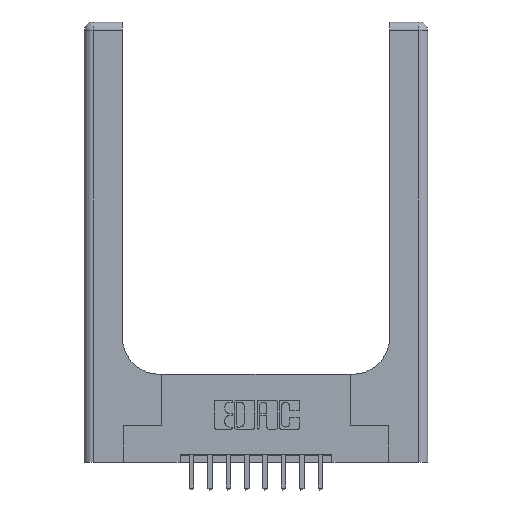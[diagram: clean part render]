
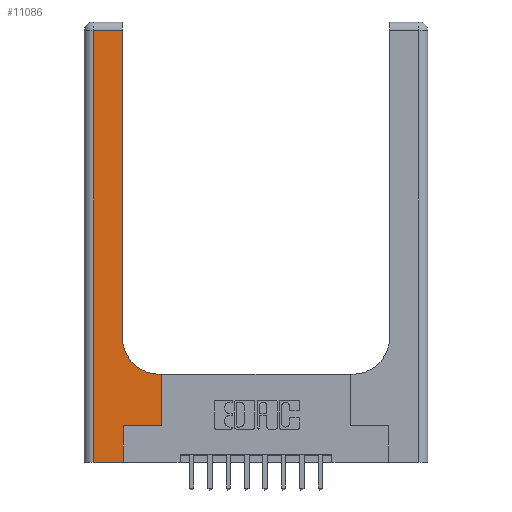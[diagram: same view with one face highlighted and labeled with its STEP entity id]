
A CAD part, top view. The second image highlights one B-rep face of the part: STEP entity #11086.
In plain terms, the highlighted planar face has unit normal (0, 0, 1).
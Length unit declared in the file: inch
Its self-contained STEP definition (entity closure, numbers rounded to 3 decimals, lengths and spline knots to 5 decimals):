
#569 = PLANE ( 'NONE',  #2759 ) ;
#762 = VECTOR ( 'NONE', #5868, 39.37008 ) ;
#809 = VECTOR ( 'NONE', #9433, 39.37008 ) ;
#1351 = EDGE_CURVE ( 'NONE', #14133, #10040, #5697, .T. ) ;
#1452 = CARTESIAN_POINT ( 'NONE',  ( 0., 2.94, 0.37 ) ) ;
#1755 = FACE_OUTER_BOUND ( 'NONE', #10992, .T. ) ;
#1768 = AXIS2_PLACEMENT_3D ( 'NONE', #4816, #14086, #13074 ) ;
#2253 = DIRECTION ( 'NONE',  ( 0., -1., 0. ) ) ;
#2340 = CARTESIAN_POINT ( 'NONE',  ( 0.528, 0.6, 0.37 ) ) ;
#2605 = DIRECTION ( 'NONE',  ( 1., 0., 0. ) ) ;
#2759 = AXIS2_PLACEMENT_3D ( 'NONE', #8673, #2910, #12300 ) ;
#2910 = DIRECTION ( 'NONE',  ( 0., 0., -1. ) ) ;
#2969 = EDGE_CURVE ( 'NONE', #3422, #8053, #11844, .T. ) ;
#3422 = VERTEX_POINT ( 'NONE', #12082 ) ;
#3600 = LINE ( 'NONE', #14030, #10732 ) ;
#3647 = VERTEX_POINT ( 'NONE', #7075 ) ;
#3779 = CARTESIAN_POINT ( 'NONE',  ( 0.265, 0., 0.37 ) ) ;
#3797 = DIRECTION ( 'NONE',  ( 0., 1., 0. ) ) ;
#3826 = LINE ( 'NONE', #6956, #762 ) ;
#4143 = ORIENTED_EDGE ( 'NONE', *, *, #14719, .T. ) ;
#4364 = VERTEX_POINT ( 'NONE', #13935 ) ;
#4365 = VECTOR ( 'NONE', #2605, 39.37008 ) ;
#4420 = VECTOR ( 'NONE', #11065, 39.37008 ) ;
#4734 = CIRCLE ( 'NONE', #1768, 0.25 ) ;
#4816 = CARTESIAN_POINT ( 'NONE',  ( 0.51, 0.85, 0.37 ) ) ;
#5697 = LINE ( 'NONE', #12212, #4420 ) ;
#5868 = DIRECTION ( 'NONE',  ( 1., 0., 0. ) ) ;
#5962 = VECTOR ( 'NONE', #11554, 39.37008 ) ;
#6536 = CARTESIAN_POINT ( 'NONE',  ( 0.26, 0.85, 0.37 ) ) ;
#6956 = CARTESIAN_POINT ( 'NONE',  ( 0., 0., 0.37 ) ) ;
#6996 = CARTESIAN_POINT ( 'NONE',  ( 0.06, 0., 0.37 ) ) ;
#7001 = EDGE_CURVE ( 'NONE', #13009, #9093, #4734, .T. ) ;
#7075 = CARTESIAN_POINT ( 'NONE',  ( 0.06, 2.94, 0.37 ) ) ;
#7145 = LINE ( 'NONE', #1452, #809 ) ;
#7663 = EDGE_CURVE ( 'NONE', #10040, #3422, #10211, .T. ) ;
#8014 = VERTEX_POINT ( 'NONE', #6996 ) ;
#8053 = VERTEX_POINT ( 'NONE', #2340 ) ;
#8249 = ORIENTED_EDGE ( 'NONE', *, *, #11984, .T. ) ;
#8530 = EDGE_CURVE ( 'NONE', #8053, #13009, #12039, .T. ) ;
#8592 = ORIENTED_EDGE ( 'NONE', *, *, #8996, .T. ) ;
#8673 = CARTESIAN_POINT ( 'NONE',  ( 0., 3., 0.37 ) ) ;
#8896 = VECTOR ( 'NONE', #12176, 39.37008 ) ;
#8937 = ORIENTED_EDGE ( 'NONE', *, *, #13460, .T. ) ;
#8996 = EDGE_CURVE ( 'NONE', #3647, #8014, #3600, .T. ) ;
#9037 = CARTESIAN_POINT ( 'NONE',  ( 0.51, 0.6, 0.37 ) ) ;
#9093 = VERTEX_POINT ( 'NONE', #6536 ) ;
#9132 = CARTESIAN_POINT ( 'NONE',  ( 0.528, 0.25, 0.37 ) ) ;
#9391 = ORIENTED_EDGE ( 'NONE', *, *, #7001, .T. ) ;
#9398 = ORIENTED_EDGE ( 'NONE', *, *, #8530, .T. ) ;
#9433 = DIRECTION ( 'NONE',  ( -1., 0., 0. ) ) ;
#9625 = ORIENTED_EDGE ( 'NONE', *, *, #7663, .T. ) ;
#9722 = LINE ( 'NONE', #10811, #11582 ) ;
#9826 = CARTESIAN_POINT ( 'NONE',  ( 0.265, 0.25, 0.37 ) ) ;
#9894 = CARTESIAN_POINT ( 'NONE',  ( 0.26, 0.6, 0.37 ) ) ;
#10040 = VERTEX_POINT ( 'NONE', #9826 ) ;
#10211 = LINE ( 'NONE', #12636, #4365 ) ;
#10732 = VECTOR ( 'NONE', #2253, 39.37008 ) ;
#10811 = CARTESIAN_POINT ( 'NONE',  ( 0.26, 3., 0.37 ) ) ;
#10992 = EDGE_LOOP ( 'NONE', ( #8937, #8249, #8592, #4143, #11490, #9625, #12267, #9398, #9391 ) ) ;
#11065 = DIRECTION ( 'NONE',  ( 0., 1., 0. ) ) ;
#11086 = ADVANCED_FACE ( 'NONE', ( #1755 ), #569, .F. ) ;
#11490 = ORIENTED_EDGE ( 'NONE', *, *, #1351, .T. ) ;
#11554 = DIRECTION ( 'NONE',  ( 0., 1., 0. ) ) ;
#11582 = VECTOR ( 'NONE', #3797, 39.37008 ) ;
#11844 = LINE ( 'NONE', #9132, #5962 ) ;
#11984 = EDGE_CURVE ( 'NONE', #4364, #3647, #7145, .T. ) ;
#12039 = LINE ( 'NONE', #9894, #8896 ) ;
#12082 = CARTESIAN_POINT ( 'NONE',  ( 0.528, 0.25, 0.37 ) ) ;
#12176 = DIRECTION ( 'NONE',  ( -1., 0., 0. ) ) ;
#12212 = CARTESIAN_POINT ( 'NONE',  ( 0.265, 0., 0.37 ) ) ;
#12267 = ORIENTED_EDGE ( 'NONE', *, *, #2969, .T. ) ;
#12300 = DIRECTION ( 'NONE',  ( -1., 0., 0. ) ) ;
#12636 = CARTESIAN_POINT ( 'NONE',  ( 0.265, 0.25, 0.37 ) ) ;
#13009 = VERTEX_POINT ( 'NONE', #9037 ) ;
#13074 = DIRECTION ( 'NONE',  ( 1., 0., 0. ) ) ;
#13460 = EDGE_CURVE ( 'NONE', #9093, #4364, #9722, .T. ) ;
#13935 = CARTESIAN_POINT ( 'NONE',  ( 0.26, 2.94, 0.37 ) ) ;
#14030 = CARTESIAN_POINT ( 'NONE',  ( 0.06, 3., 0.37 ) ) ;
#14086 = DIRECTION ( 'NONE',  ( 0., 0., -1. ) ) ;
#14133 = VERTEX_POINT ( 'NONE', #3779 ) ;
#14719 = EDGE_CURVE ( 'NONE', #8014, #14133, #3826, .T. ) ;
